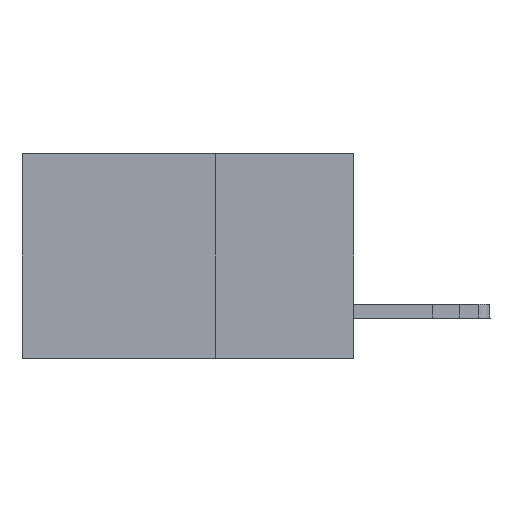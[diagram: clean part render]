
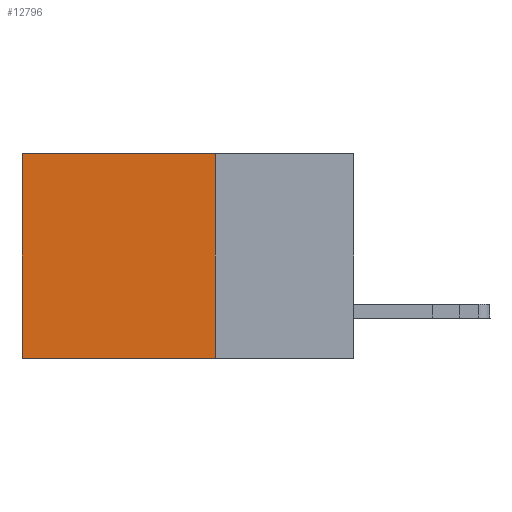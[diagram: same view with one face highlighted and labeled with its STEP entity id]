
A CAD part, left-side view. The second image highlights one B-rep face of the part: STEP entity #12796.
In plain terms, the highlighted planar face has unit normal (-1, 0, 0).
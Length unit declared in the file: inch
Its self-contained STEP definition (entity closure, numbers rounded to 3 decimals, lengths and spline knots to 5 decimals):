
#408 = DIRECTION ( 'NONE',  ( 0., 0., -1. ) ) ;
#588 = FACE_OUTER_BOUND ( 'NONE', #1374, .T. ) ;
#1172 = LINE ( 'NONE', #7369, #10477 ) ;
#1260 = VERTEX_POINT ( 'NONE', #14116 ) ;
#1299 = VERTEX_POINT ( 'NONE', #13716 ) ;
#1374 = EDGE_LOOP ( 'NONE', ( #10419, #3349, #18721, #8795 ) ) ;
#1717 = LINE ( 'NONE', #8776, #9983 ) ;
#2826 = VECTOR ( 'NONE', #408, 39.37008 ) ;
#3020 = AXIS2_PLACEMENT_3D ( 'NONE', #8989, #15765, #5960 ) ;
#3349 = ORIENTED_EDGE ( 'NONE', *, *, #9146, .F. ) ;
#3594 = VERTEX_POINT ( 'NONE', #8816 ) ;
#5137 = VERTEX_POINT ( 'NONE', #17115 ) ;
#5960 = DIRECTION ( 'NONE',  ( 0., 0., -1. ) ) ;
#7220 = PLANE ( 'NONE',  #3020 ) ;
#7246 = EDGE_CURVE ( 'NONE', #3594, #5137, #11566, .T. ) ;
#7369 = CARTESIAN_POINT ( 'NONE',  ( 0.2875, 0.25, 0. ) ) ;
#8776 = CARTESIAN_POINT ( 'NONE',  ( 0.2875, 0.25, -0.37 ) ) ;
#8795 = ORIENTED_EDGE ( 'NONE', *, *, #21030, .T. ) ;
#8816 = CARTESIAN_POINT ( 'NONE',  ( 0.2875, 0.25, 0. ) ) ;
#8989 = CARTESIAN_POINT ( 'NONE',  ( 0.2875, 0.25, 0. ) ) ;
#9146 = EDGE_CURVE ( 'NONE', #5137, #1299, #1717, .T. ) ;
#9983 = VECTOR ( 'NONE', #10451, 39.37008 ) ;
#10238 = CARTESIAN_POINT ( 'NONE',  ( 0.2875, 0.25, 0. ) ) ;
#10419 = ORIENTED_EDGE ( 'NONE', *, *, #13125, .T. ) ;
#10451 = DIRECTION ( 'NONE',  ( 0., 1., 0. ) ) ;
#10477 = VECTOR ( 'NONE', #10721, 39.37008 ) ;
#10721 = DIRECTION ( 'NONE',  ( 0., 1., 0. ) ) ;
#11566 = LINE ( 'NONE', #10238, #2826 ) ;
#11869 = LINE ( 'NONE', #18059, #20373 ) ;
#12796 = ADVANCED_FACE ( 'NONE', ( #588 ), #7220, .F. ) ;
#13125 = EDGE_CURVE ( 'NONE', #1260, #1299, #11869, .T. ) ;
#13293 = DIRECTION ( 'NONE',  ( 0., 0., -1. ) ) ;
#13716 = CARTESIAN_POINT ( 'NONE',  ( 0.2875, 0.6, -0.37 ) ) ;
#14116 = CARTESIAN_POINT ( 'NONE',  ( 0.2875, 0.6, 0. ) ) ;
#15765 = DIRECTION ( 'NONE',  ( 1., 0., 0. ) ) ;
#17115 = CARTESIAN_POINT ( 'NONE',  ( 0.2875, 0.25, -0.37 ) ) ;
#18059 = CARTESIAN_POINT ( 'NONE',  ( 0.2875, 0.6, 0. ) ) ;
#18721 = ORIENTED_EDGE ( 'NONE', *, *, #7246, .F. ) ;
#20373 = VECTOR ( 'NONE', #13293, 39.37008 ) ;
#21030 = EDGE_CURVE ( 'NONE', #3594, #1260, #1172, .T. ) ;
